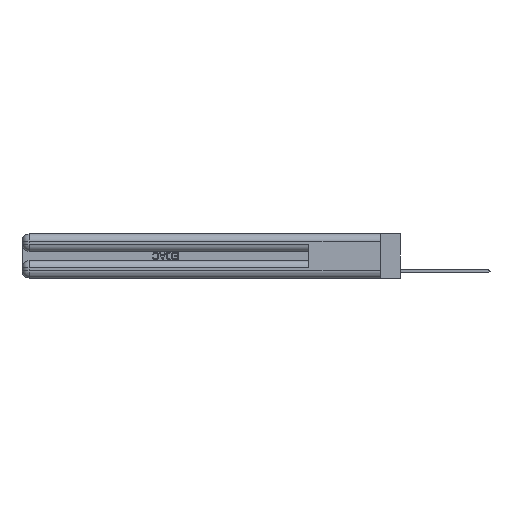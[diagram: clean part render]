
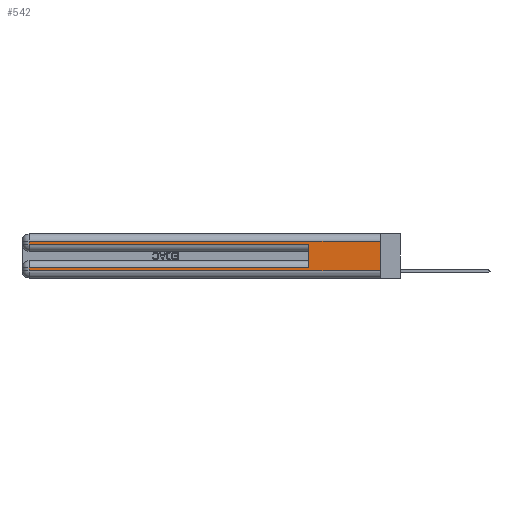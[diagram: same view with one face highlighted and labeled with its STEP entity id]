
A CAD part, left-side view. The second image highlights one B-rep face of the part: STEP entity #542.
In plain terms, the highlighted planar face has unit normal (-1, 0, 0).
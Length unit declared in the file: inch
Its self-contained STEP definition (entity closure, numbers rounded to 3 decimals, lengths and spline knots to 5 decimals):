
#69 = DIRECTION ( 'NONE',  ( 0., 1., 0. ) ) ;
#193 = EDGE_CURVE ( 'NONE', #17759, #24873, #9609, .T. ) ;
#407 = CARTESIAN_POINT ( 'NONE',  ( 0., 0.6, 0.285 ) ) ;
#542 = ADVANCED_FACE ( 'NONE', ( #22469 ), #2207, .F. ) ;
#1294 = ORIENTED_EDGE ( 'NONE', *, *, #26114, .T. ) ;
#1878 = EDGE_CURVE ( 'NONE', #8870, #24873, #7850, .T. ) ;
#1884 = VERTEX_POINT ( 'NONE', #26629 ) ;
#1980 = VECTOR ( 'NONE', #9583, 39.37008 ) ;
#2207 = PLANE ( 'NONE',  #30786 ) ;
#2581 = ORIENTED_EDGE ( 'NONE', *, *, #28399, .T. ) ;
#3974 = VERTEX_POINT ( 'NONE', #25547 ) ;
#4440 = EDGE_LOOP ( 'NONE', ( #28269, #24147, #2581, #5395, #27799, #8904, #1294, #19353 ) ) ;
#4496 = CARTESIAN_POINT ( 'NONE',  ( 0., 0., 0.37 ) ) ;
#5395 = ORIENTED_EDGE ( 'NONE', *, *, #193, .T. ) ;
#6915 = CARTESIAN_POINT ( 'NONE',  ( 0., 0., 0.085 ) ) ;
#7129 = VECTOR ( 'NONE', #69, 39.37008 ) ;
#7850 = LINE ( 'NONE', #21592, #1980 ) ;
#7870 = VECTOR ( 'NONE', #26110, 39.37008 ) ;
#8870 = VERTEX_POINT ( 'NONE', #25615 ) ;
#8904 = ORIENTED_EDGE ( 'NONE', *, *, #17896, .T. ) ;
#9034 = VERTEX_POINT ( 'NONE', #30743 ) ;
#9077 = LINE ( 'NONE', #6915, #21593 ) ;
#9164 = LINE ( 'NONE', #29509, #16195 ) ;
#9426 = EDGE_CURVE ( 'NONE', #9034, #1884, #12913, .T. ) ;
#9583 = DIRECTION ( 'NONE',  ( 0., 0., 1. ) ) ;
#9609 = LINE ( 'NONE', #26008, #26389 ) ;
#9899 = DIRECTION ( 'NONE',  ( 1., 0., 0. ) ) ;
#10222 = LINE ( 'NONE', #12639, #30526 ) ;
#11799 = CARTESIAN_POINT ( 'NONE',  ( 0., 2.94, 0.285 ) ) ;
#12639 = CARTESIAN_POINT ( 'NONE',  ( 0., 2.94, 0.37 ) ) ;
#12913 = LINE ( 'NONE', #22535, #24311 ) ;
#13440 = DIRECTION ( 'NONE',  ( 0., -1., 0. ) ) ;
#14502 = LINE ( 'NONE', #18267, #7870 ) ;
#15372 = DIRECTION ( 'NONE',  ( 0., 0., -1. ) ) ;
#15752 = LINE ( 'NONE', #19129, #7129 ) ;
#16195 = VECTOR ( 'NONE', #18194, 39.37008 ) ;
#17100 = DIRECTION ( 'NONE',  ( 0., 1., 0. ) ) ;
#17759 = VERTEX_POINT ( 'NONE', #11799 ) ;
#17896 = EDGE_CURVE ( 'NONE', #8870, #21849, #9077, .T. ) ;
#18194 = DIRECTION ( 'NONE',  ( 0., 0., -1. ) ) ;
#18267 = CARTESIAN_POINT ( 'NONE',  ( 0., 2.94, 0.37 ) ) ;
#19129 = CARTESIAN_POINT ( 'NONE',  ( 0., 0., 0.31 ) ) ;
#19353 = ORIENTED_EDGE ( 'NONE', *, *, #9426, .T. ) ;
#21592 = CARTESIAN_POINT ( 'NONE',  ( 0., 0.6, 0.145 ) ) ;
#21593 = VECTOR ( 'NONE', #17100, 39.37008 ) ;
#21849 = VERTEX_POINT ( 'NONE', #30096 ) ;
#22469 = FACE_OUTER_BOUND ( 'NONE', #4440, .T. ) ;
#22535 = CARTESIAN_POINT ( 'NONE',  ( 0., 0., 0.06 ) ) ;
#24147 = ORIENTED_EDGE ( 'NONE', *, *, #25250, .T. ) ;
#24311 = VECTOR ( 'NONE', #25272, 39.37008 ) ;
#24873 = VERTEX_POINT ( 'NONE', #407 ) ;
#25250 = EDGE_CURVE ( 'NONE', #26825, #3974, #15752, .T. ) ;
#25272 = DIRECTION ( 'NONE',  ( 0., -1., 0. ) ) ;
#25547 = CARTESIAN_POINT ( 'NONE',  ( 0., 2.94, 0.31 ) ) ;
#25615 = CARTESIAN_POINT ( 'NONE',  ( 0., 0.6, 0.085 ) ) ;
#26008 = CARTESIAN_POINT ( 'NONE',  ( 0., 0., 0.285 ) ) ;
#26110 = DIRECTION ( 'NONE',  ( 0., 0., -1. ) ) ;
#26114 = EDGE_CURVE ( 'NONE', #21849, #9034, #14502, .T. ) ;
#26389 = VECTOR ( 'NONE', #13440, 39.37008 ) ;
#26629 = CARTESIAN_POINT ( 'NONE',  ( 0., 0., 0.06 ) ) ;
#26825 = VERTEX_POINT ( 'NONE', #28356 ) ;
#27351 = DIRECTION ( 'NONE',  ( 0., 0., -1. ) ) ;
#27799 = ORIENTED_EDGE ( 'NONE', *, *, #1878, .F. ) ;
#28269 = ORIENTED_EDGE ( 'NONE', *, *, #32046, .F. ) ;
#28356 = CARTESIAN_POINT ( 'NONE',  ( 0., 0., 0.31 ) ) ;
#28399 = EDGE_CURVE ( 'NONE', #3974, #17759, #10222, .T. ) ;
#29509 = CARTESIAN_POINT ( 'NONE',  ( 0., 0., 0.37 ) ) ;
#30096 = CARTESIAN_POINT ( 'NONE',  ( 0., 2.94, 0.085 ) ) ;
#30526 = VECTOR ( 'NONE', #15372, 39.37008 ) ;
#30743 = CARTESIAN_POINT ( 'NONE',  ( 0., 2.94, 0.06 ) ) ;
#30786 = AXIS2_PLACEMENT_3D ( 'NONE', #4496, #9899, #27351 ) ;
#32046 = EDGE_CURVE ( 'NONE', #26825, #1884, #9164, .T. ) ;
